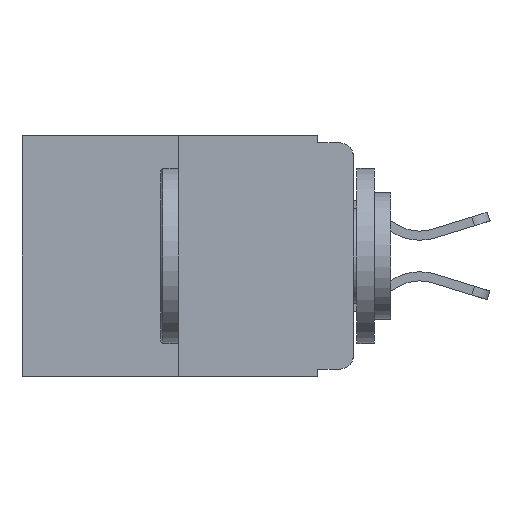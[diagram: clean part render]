
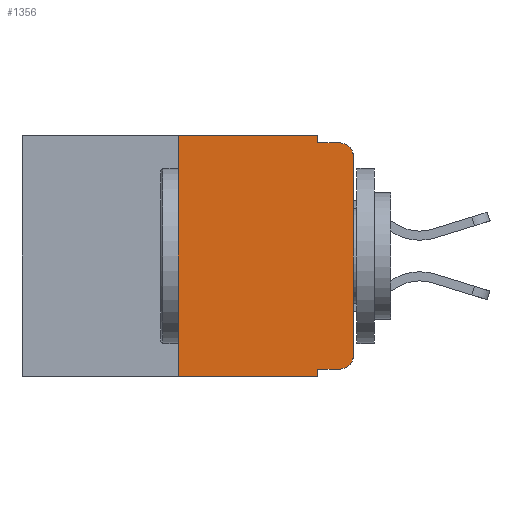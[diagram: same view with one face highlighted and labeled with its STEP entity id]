
A CAD part, left-side view. The second image highlights one B-rep face of the part: STEP entity #1356.
In plain terms, the highlighted planar face has unit normal (-1, 0, 0).
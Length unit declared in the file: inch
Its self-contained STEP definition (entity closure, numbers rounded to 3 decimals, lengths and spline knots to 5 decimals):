
#150 = DIRECTION ( 'NONE',  ( 0., 0., -1. ) ) ;
#271 = EDGE_CURVE ( 'NONE', #9019, #602, #490, .T. ) ;
#490 = LINE ( 'NONE', #7117, #3670 ) ;
#528 = DIRECTION ( 'NONE',  ( 0., 0., -1. ) ) ;
#552 = CARTESIAN_POINT ( 'NONE',  ( 0., 0.25, 0. ) ) ;
#602 = VERTEX_POINT ( 'NONE', #7868 ) ;
#650 = FACE_OUTER_BOUND ( 'NONE', #11194, .T. ) ;
#711 = VECTOR ( 'NONE', #8484, 39.37008 ) ;
#806 = VERTEX_POINT ( 'NONE', #9318 ) ;
#829 = VERTEX_POINT ( 'NONE', #4524 ) ;
#857 = CARTESIAN_POINT ( 'NONE',  ( 0., 0.02, -0.313 ) ) ;
#972 = ORIENTED_EDGE ( 'NONE', *, *, #271, .T. ) ;
#1013 = DIRECTION ( 'NONE',  ( 0., -1., 0. ) ) ;
#1070 = EDGE_CURVE ( 'NONE', #602, #829, #1904, .T. ) ;
#1092 = LINE ( 'NONE', #7642, #9189 ) ;
#1151 = AXIS2_PLACEMENT_3D ( 'NONE', #3579, #6314, #528 ) ;
#1237 = ORIENTED_EDGE ( 'NONE', *, *, #4457, .T. ) ;
#1356 = ADVANCED_FACE ( 'NONE', ( #650 ), #5326, .F. ) ;
#1458 = VECTOR ( 'NONE', #1013, 39.37008 ) ;
#1783 = ORIENTED_EDGE ( 'NONE', *, *, #3341, .F. ) ;
#1886 = LINE ( 'NONE', #8761, #1458 ) ;
#1904 = CIRCLE ( 'NONE', #2113, 0.02 ) ;
#1946 = VECTOR ( 'NONE', #8013, 39.37008 ) ;
#2113 = AXIS2_PLACEMENT_3D ( 'NONE', #857, #12487, #150 ) ;
#2410 = DIRECTION ( 'NONE',  ( 0., -1., 0. ) ) ;
#2642 = DIRECTION ( 'NONE',  ( -1., 0., 0. ) ) ;
#2766 = CARTESIAN_POINT ( 'NONE',  ( 0., 0.051, -0.343 ) ) ;
#2811 = CARTESIAN_POINT ( 'NONE',  ( 0., 0.051, 0. ) ) ;
#2948 = VECTOR ( 'NONE', #3754, 39.37008 ) ;
#3220 = VERTEX_POINT ( 'NONE', #10859 ) ;
#3341 = EDGE_CURVE ( 'NONE', #7850, #10647, #1886, .T. ) ;
#3579 = CARTESIAN_POINT ( 'NONE',  ( 0., 0.473, 0. ) ) ;
#3606 = CARTESIAN_POINT ( 'NONE',  ( 0., 0.02, -0.03 ) ) ;
#3670 = VECTOR ( 'NONE', #8957, 39.37008 ) ;
#3754 = DIRECTION ( 'NONE',  ( 0., -1., 0. ) ) ;
#4055 = DIRECTION ( 'NONE',  ( 0., 0., 1. ) ) ;
#4105 = CARTESIAN_POINT ( 'NONE',  ( 0., 0., 0. ) ) ;
#4381 = VECTOR ( 'NONE', #2410, 39.37008 ) ;
#4457 = EDGE_CURVE ( 'NONE', #829, #3220, #9706, .T. ) ;
#4524 = CARTESIAN_POINT ( 'NONE',  ( 0., 0., -0.313 ) ) ;
#4610 = VERTEX_POINT ( 'NONE', #552 ) ;
#4634 = LINE ( 'NONE', #2811, #711 ) ;
#4910 = DIRECTION ( 'NONE',  ( 0., 0., 1. ) ) ;
#5299 = VECTOR ( 'NONE', #4910, 39.37008 ) ;
#5326 = PLANE ( 'NONE',  #1151 ) ;
#6016 = VERTEX_POINT ( 'NONE', #2766 ) ;
#6043 = CARTESIAN_POINT ( 'NONE',  ( 0., 0.051, -0.333 ) ) ;
#6128 = ORIENTED_EDGE ( 'NONE', *, *, #7065, .T. ) ;
#6314 = DIRECTION ( 'NONE',  ( 1., 0., 0. ) ) ;
#6462 = VERTEX_POINT ( 'NONE', #11012 ) ;
#6468 = DIRECTION ( 'NONE',  ( 0., 0., -1. ) ) ;
#6519 = EDGE_CURVE ( 'NONE', #9019, #6016, #4634, .T. ) ;
#6672 = ORIENTED_EDGE ( 'NONE', *, *, #1070, .T. ) ;
#6762 = CARTESIAN_POINT ( 'NONE',  ( 0., 0.473, -0.343 ) ) ;
#7002 = CARTESIAN_POINT ( 'NONE',  ( 0., 0.051, 0. ) ) ;
#7065 = EDGE_CURVE ( 'NONE', #6462, #6016, #8717, .T. ) ;
#7103 = CARTESIAN_POINT ( 'NONE',  ( 0., 0.02, -0.01 ) ) ;
#7113 = CARTESIAN_POINT ( 'NONE',  ( 0., 0.473, 0. ) ) ;
#7117 = CARTESIAN_POINT ( 'NONE',  ( 0., 0.051, -0.333 ) ) ;
#7245 = LINE ( 'NONE', #7002, #1946 ) ;
#7360 = ORIENTED_EDGE ( 'NONE', *, *, #6519, .F. ) ;
#7642 = CARTESIAN_POINT ( 'NONE',  ( 0., 0.25, 0. ) ) ;
#7850 = VERTEX_POINT ( 'NONE', #10207 ) ;
#7868 = CARTESIAN_POINT ( 'NONE',  ( 0., 0.02, -0.333 ) ) ;
#7917 = EDGE_CURVE ( 'NONE', #3220, #10647, #11526, .T. ) ;
#8013 = DIRECTION ( 'NONE',  ( 0., 0., -1. ) ) ;
#8394 = ORIENTED_EDGE ( 'NONE', *, *, #10165, .F. ) ;
#8484 = DIRECTION ( 'NONE',  ( 0., 0., -1. ) ) ;
#8717 = LINE ( 'NONE', #6762, #2948 ) ;
#8761 = CARTESIAN_POINT ( 'NONE',  ( 0., 0.051, -0.01 ) ) ;
#8957 = DIRECTION ( 'NONE',  ( 0., -1., 0. ) ) ;
#9019 = VERTEX_POINT ( 'NONE', #6043 ) ;
#9109 = ORIENTED_EDGE ( 'NONE', *, *, #7917, .T. ) ;
#9189 = VECTOR ( 'NONE', #4055, 39.37008 ) ;
#9318 = CARTESIAN_POINT ( 'NONE',  ( 0., 0.051, 0. ) ) ;
#9438 = ORIENTED_EDGE ( 'NONE', *, *, #10044, .F. ) ;
#9706 = LINE ( 'NONE', #4105, #5299 ) ;
#10044 = EDGE_CURVE ( 'NONE', #6462, #4610, #1092, .T. ) ;
#10165 = EDGE_CURVE ( 'NONE', #806, #7850, #7245, .T. ) ;
#10207 = CARTESIAN_POINT ( 'NONE',  ( 0., 0.051, -0.01 ) ) ;
#10316 = ORIENTED_EDGE ( 'NONE', *, *, #11754, .F. ) ;
#10647 = VERTEX_POINT ( 'NONE', #7103 ) ;
#10859 = CARTESIAN_POINT ( 'NONE',  ( 0., 0., -0.03 ) ) ;
#11012 = CARTESIAN_POINT ( 'NONE',  ( 0., 0.25, -0.343 ) ) ;
#11123 = AXIS2_PLACEMENT_3D ( 'NONE', #3606, #2642, #6468 ) ;
#11194 = EDGE_LOOP ( 'NONE', ( #1237, #9109, #1783, #8394, #10316, #9438, #6128, #7360, #972, #6672 ) ) ;
#11526 = CIRCLE ( 'NONE', #11123, 0.02 ) ;
#11754 = EDGE_CURVE ( 'NONE', #4610, #806, #11863, .T. ) ;
#11863 = LINE ( 'NONE', #7113, #4381 ) ;
#12487 = DIRECTION ( 'NONE',  ( -1., 0., 0. ) ) ;
